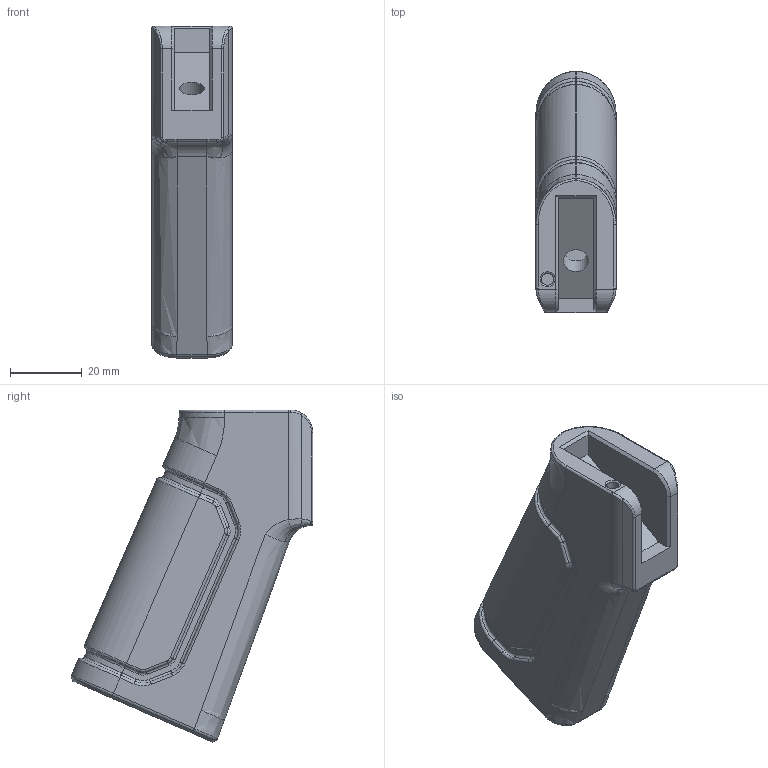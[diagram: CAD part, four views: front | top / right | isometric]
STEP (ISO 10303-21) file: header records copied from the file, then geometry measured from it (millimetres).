
FILE_DESCRIPTION(/* description */ (''),/* implementation_level */ '2;1');
FILE_NAME(/* name */ 'Mini Grip.step',/* time_stamp */ '2021-03-04T07:46:51-05:00',/* author */ (''),/* organization */ (''),/* preprocessor_version */ 'ST-DEVELOPER v18.1',/* originating_system */ 'Autodesk Translation Framework v9.7.1.1290',/* authorisation */ '');
FILE_SCHEMA (('AUTOMOTIVE_DESIGN { 1 0 10303 214 3 1 1 }'));
Length unit declared in the file: millimetre
Products named in the file (1): Mini Grip
Bounding box: 22.33 x 67.19 x 92.34 mm (x, y, z)
Volume: 45619.8 mm3; surface area: 18469.4 mm2
Topology: 1 solids, 1 shells, 304 faces, 719 edges, 415 vertices
Faces by surface type: bspline 124, cylinder 96, plane 52, torus 25, cone 7
Full cylindrical faces by diameter (mm): 3.4 x1, 7 x1
Entity records: 14277 total; most frequent: CARTESIAN_POINT 7899, ORIENTED_EDGE 1430, DIRECTION 1143, EDGE_CURVE 715, AXIS2_PLACEMENT_3D 439, VERTEX_POINT 415, EDGE_LOOP 308, FACE_OUTER_BOUND 304
